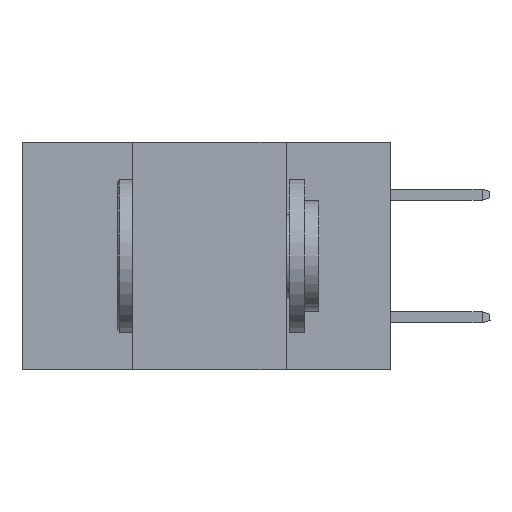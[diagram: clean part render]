
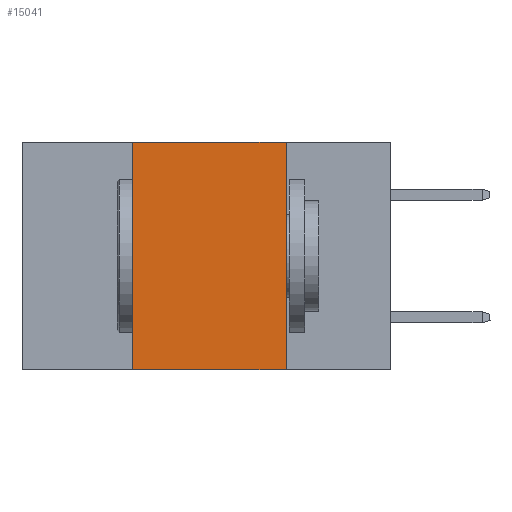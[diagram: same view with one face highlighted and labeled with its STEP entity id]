
A CAD part, left-side view. The second image highlights one B-rep face of the part: STEP entity #15041.
In plain terms, the highlighted planar face has unit normal (-1, 0, 0).
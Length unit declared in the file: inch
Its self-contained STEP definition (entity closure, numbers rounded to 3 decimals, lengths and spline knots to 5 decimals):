
#1236 = CARTESIAN_POINT ( 'NONE',  ( 0., 0.6, 0. ) ) ;
#1948 = VERTEX_POINT ( 'NONE', #17997 ) ;
#2389 = ORIENTED_EDGE ( 'NONE', *, *, #14362, .F. ) ;
#2760 = DIRECTION ( 'NONE',  ( 1., 0., 0. ) ) ;
#2885 = PLANE ( 'NONE',  #15605 ) ;
#2991 = VECTOR ( 'NONE', #7239, 39.37008 ) ;
#3015 = VERTEX_POINT ( 'NONE', #12873 ) ;
#3027 = LINE ( 'NONE', #17725, #17393 ) ;
#4952 = EDGE_CURVE ( 'NONE', #8723, #1948, #10016, .T. ) ;
#5365 = CARTESIAN_POINT ( 'NONE',  ( 0., 0.42, -0.37 ) ) ;
#5605 = DIRECTION ( 'NONE',  ( 0., 0., 1. ) ) ;
#6325 = DIRECTION ( 'NONE',  ( 0., -1., 0. ) ) ;
#7239 = DIRECTION ( 'NONE',  ( 0., 0., -1. ) ) ;
#8604 = LINE ( 'NONE', #12643, #10006 ) ;
#8692 = CARTESIAN_POINT ( 'NONE',  ( 0., 0.17, 0. ) ) ;
#8723 = VERTEX_POINT ( 'NONE', #8692 ) ;
#9445 = ORIENTED_EDGE ( 'NONE', *, *, #11090, .T. ) ;
#10006 = VECTOR ( 'NONE', #12505, 39.37008 ) ;
#10016 = LINE ( 'NONE', #16293, #2991 ) ;
#10617 = CARTESIAN_POINT ( 'NONE',  ( 0., 0.6, -0.37 ) ) ;
#11077 = LINE ( 'NONE', #10617, #14157 ) ;
#11090 = EDGE_CURVE ( 'NONE', #12659, #1948, #11077, .T. ) ;
#12505 = DIRECTION ( 'NONE',  ( 0., -1., 0. ) ) ;
#12643 = CARTESIAN_POINT ( 'NONE',  ( 0., 0.6, 0. ) ) ;
#12659 = VERTEX_POINT ( 'NONE', #5365 ) ;
#12873 = CARTESIAN_POINT ( 'NONE',  ( 0., 0.42, 0. ) ) ;
#13376 = EDGE_CURVE ( 'NONE', #12659, #3015, #3027, .T. ) ;
#14157 = VECTOR ( 'NONE', #6325, 39.37008 ) ;
#14362 = EDGE_CURVE ( 'NONE', #3015, #8723, #8604, .T. ) ;
#14514 = FACE_OUTER_BOUND ( 'NONE', #18665, .T. ) ;
#14693 = ORIENTED_EDGE ( 'NONE', *, *, #4952, .F. ) ;
#14889 = ORIENTED_EDGE ( 'NONE', *, *, #13376, .F. ) ;
#15041 = ADVANCED_FACE ( 'NONE', ( #14514 ), #2885, .F. ) ;
#15605 = AXIS2_PLACEMENT_3D ( 'NONE', #1236, #2760, #17958 ) ;
#16293 = CARTESIAN_POINT ( 'NONE',  ( 0., 0.17, 0. ) ) ;
#17393 = VECTOR ( 'NONE', #5605, 39.37008 ) ;
#17725 = CARTESIAN_POINT ( 'NONE',  ( 0., 0.42, 0. ) ) ;
#17958 = DIRECTION ( 'NONE',  ( 0., 0., -1. ) ) ;
#17997 = CARTESIAN_POINT ( 'NONE',  ( 0., 0.17, -0.37 ) ) ;
#18665 = EDGE_LOOP ( 'NONE', ( #14693, #2389, #14889, #9445 ) ) ;
